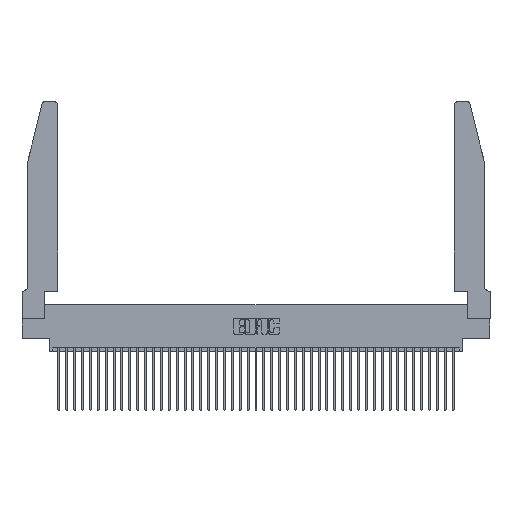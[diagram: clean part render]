
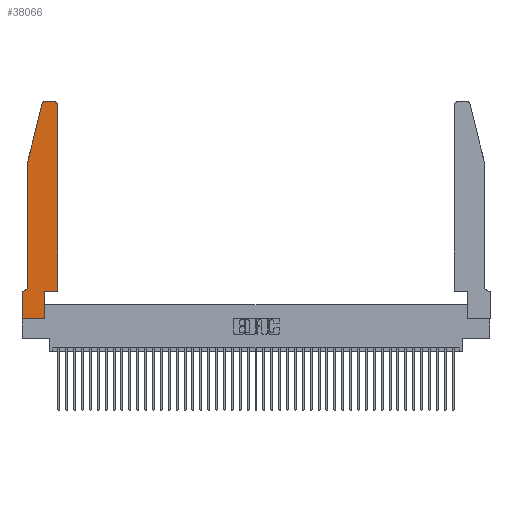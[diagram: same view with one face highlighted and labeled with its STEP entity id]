
A CAD part, top view. The second image highlights one B-rep face of the part: STEP entity #38066.
In plain terms, the highlighted planar face has unit normal (0, 0, 1).
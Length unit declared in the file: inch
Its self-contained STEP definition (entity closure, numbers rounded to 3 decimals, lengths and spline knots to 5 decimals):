
#344 = DIRECTION ( 'NONE',  ( 1., 0., 0. ) ) ;
#655 = VERTEX_POINT ( 'NONE', #27493 ) ;
#808 = VERTEX_POINT ( 'NONE', #23165 ) ;
#838 = CARTESIAN_POINT ( 'NONE',  ( 0.0055, 0.35, 0.37 ) ) ;
#1015 = EDGE_CURVE ( 'NONE', #15155, #16034, #19048, .T. ) ;
#1207 = CARTESIAN_POINT ( 'NONE',  ( 0.2605, 2.75, 0.37 ) ) ;
#1279 = VERTEX_POINT ( 'NONE', #5103 ) ;
#1773 = CARTESIAN_POINT ( 'NONE',  ( 0.284, 2.75, 0.37 ) ) ;
#2813 = EDGE_CURVE ( 'NONE', #16034, #808, #14678, .T. ) ;
#3134 = VERTEX_POINT ( 'NONE', #838 ) ;
#3527 = LINE ( 'NONE', #32728, #4634 ) ;
#4035 = CARTESIAN_POINT ( 'NONE',  ( 0.4205, 2.72, 0.37 ) ) ;
#4056 = LINE ( 'NONE', #37252, #11062 ) ;
#4232 = VERTEX_POINT ( 'NONE', #1773 ) ;
#4634 = VECTOR ( 'NONE', #9060, 39.37008 ) ;
#5055 = ORIENTED_EDGE ( 'NONE', *, *, #42771, .T. ) ;
#5103 = CARTESIAN_POINT ( 'NONE',  ( 0.4505, 0.35, 0.37 ) ) ;
#5328 = AXIS2_PLACEMENT_3D ( 'NONE', #7222, #20881, #344 ) ;
#6149 = VECTOR ( 'NONE', #42377, 39.37008 ) ;
#7222 = CARTESIAN_POINT ( 'NONE',  ( 0., 0.35, 0.37 ) ) ;
#7456 = EDGE_CURVE ( 'NONE', #41823, #11102, #25633, .T. ) ;
#7550 = DIRECTION ( 'NONE',  ( 1., 0., 0. ) ) ;
#8042 = AXIS2_PLACEMENT_3D ( 'NONE', #4035, #27740, #7550 ) ;
#8118 = CARTESIAN_POINT ( 'NONE',  ( 0.2865, 0.35, 0.37 ) ) ;
#8283 = FACE_OUTER_BOUND ( 'NONE', #43312, .T. ) ;
#8326 = ORIENTED_EDGE ( 'NONE', *, *, #26272, .T. ) ;
#8571 = ORIENTED_EDGE ( 'NONE', *, *, #2813, .T. ) ;
#9060 = DIRECTION ( 'NONE',  ( 0., 1., 0. ) ) ;
#9085 = CARTESIAN_POINT ( 'NONE',  ( 0., 0., 0.37 ) ) ;
#9821 = LINE ( 'NONE', #21708, #35583 ) ;
#10129 = VERTEX_POINT ( 'NONE', #19170 ) ;
#10695 = CARTESIAN_POINT ( 'NONE',  ( 0.2865, 0., 0.37 ) ) ;
#11062 = VECTOR ( 'NONE', #40607, 39.37008 ) ;
#11102 = VERTEX_POINT ( 'NONE', #10695 ) ;
#12475 = LINE ( 'NONE', #8118, #13531 ) ;
#13531 = VECTOR ( 'NONE', #41724, 39.37008 ) ;
#14416 = ORIENTED_EDGE ( 'NONE', *, *, #18797, .T. ) ;
#14678 = LINE ( 'NONE', #36544, #41377 ) ;
#15155 = VERTEX_POINT ( 'NONE', #40575 ) ;
#15384 = EDGE_CURVE ( 'NONE', #11102, #655, #12475, .T. ) ;
#15689 = DIRECTION ( 'NONE',  ( 0., 0., -1. ) ) ;
#16034 = VERTEX_POINT ( 'NONE', #35415 ) ;
#18371 = CARTESIAN_POINT ( 'NONE',  ( 0.284, 2.72, 0.37 ) ) ;
#18488 = ORIENTED_EDGE ( 'NONE', *, *, #7456, .T. ) ;
#18797 = EDGE_CURVE ( 'NONE', #4232, #15155, #30576, .T. ) ;
#18809 = EDGE_CURVE ( 'NONE', #23885, #4232, #21705, .T. ) ;
#19048 = LINE ( 'NONE', #39644, #43496 ) ;
#19170 = CARTESIAN_POINT ( 'NONE',  ( 0., 0.35, 0.37 ) ) ;
#20881 = DIRECTION ( 'NONE',  ( 0., 0., 1. ) ) ;
#21597 = ORIENTED_EDGE ( 'NONE', *, *, #15384, .T. ) ;
#21697 = DIRECTION ( 'NONE',  ( 1., 0., 0. ) ) ;
#21705 = LINE ( 'NONE', #1207, #29538 ) ;
#21708 = CARTESIAN_POINT ( 'NONE',  ( 0.0755, 0.35, 0.37 ) ) ;
#21833 = EDGE_CURVE ( 'NONE', #808, #3134, #27213, .T. ) ;
#22579 = ORIENTED_EDGE ( 'NONE', *, *, #32220, .T. ) ;
#23165 = CARTESIAN_POINT ( 'NONE',  ( 0.0755, 0.42, 0.37 ) ) ;
#23885 = VERTEX_POINT ( 'NONE', #39431 ) ;
#25067 = DIRECTION ( 'NONE',  ( -1., 0., 0. ) ) ;
#25213 = LINE ( 'NONE', #42238, #6149 ) ;
#25633 = LINE ( 'NONE', #38494, #34489 ) ;
#25707 = ORIENTED_EDGE ( 'NONE', *, *, #31964, .T. ) ;
#26256 = ORIENTED_EDGE ( 'NONE', *, *, #21833, .T. ) ;
#26272 = EDGE_CURVE ( 'NONE', #10129, #41823, #25213, .T. ) ;
#27213 = CIRCLE ( 'NONE', #32574, 0.07 ) ;
#27493 = CARTESIAN_POINT ( 'NONE',  ( 0.2865, 0.35, 0.37 ) ) ;
#27740 = DIRECTION ( 'NONE',  ( 0., 0., 1. ) ) ;
#28253 = DIRECTION ( 'NONE',  ( -1., 0., 0. ) ) ;
#29538 = VECTOR ( 'NONE', #28253, 39.37008 ) ;
#29832 = DIRECTION ( 'NONE',  ( 0., -1., 0. ) ) ;
#30576 = CIRCLE ( 'NONE', #42296, 0.03 ) ;
#30964 = DIRECTION ( 'NONE',  ( -0.239, -0.971, 0. ) ) ;
#31203 = ORIENTED_EDGE ( 'NONE', *, *, #18809, .T. ) ;
#31964 = EDGE_CURVE ( 'NONE', #1279, #41457, #3527, .T. ) ;
#32220 = EDGE_CURVE ( 'NONE', #655, #1279, #4056, .T. ) ;
#32574 = AXIS2_PLACEMENT_3D ( 'NONE', #35705, #15689, #39066 ) ;
#32728 = CARTESIAN_POINT ( 'NONE',  ( 0.4505, 0.35, 0.37 ) ) ;
#34323 = ORIENTED_EDGE ( 'NONE', *, *, #1015, .T. ) ;
#34489 = VECTOR ( 'NONE', #41820, 39.37008 ) ;
#34770 = EDGE_CURVE ( 'NONE', #3134, #10129, #9821, .T. ) ;
#35415 = CARTESIAN_POINT ( 'NONE',  ( 0.0755, 2., 0.37 ) ) ;
#35583 = VECTOR ( 'NONE', #25067, 39.37008 ) ;
#35705 = CARTESIAN_POINT ( 'NONE',  ( 0.0055, 0.42, 0.37 ) ) ;
#36544 = CARTESIAN_POINT ( 'NONE',  ( 0.0755, 2., 0.37 ) ) ;
#37252 = CARTESIAN_POINT ( 'NONE',  ( 0.4505, 0.35, 0.37 ) ) ;
#38066 = ADVANCED_FACE ( 'NONE', ( #8283 ), #40717, .T. ) ;
#38494 = CARTESIAN_POINT ( 'NONE',  ( 0., 0., 0.37 ) ) ;
#39066 = DIRECTION ( 'NONE',  ( -1., 0., 0. ) ) ;
#39431 = CARTESIAN_POINT ( 'NONE',  ( 0.4205, 2.75, 0.37 ) ) ;
#39644 = CARTESIAN_POINT ( 'NONE',  ( 0.0755, 2., 0.37 ) ) ;
#40575 = CARTESIAN_POINT ( 'NONE',  ( 0.25487, 2.72718, 0.37 ) ) ;
#40607 = DIRECTION ( 'NONE',  ( 1., 0., 0. ) ) ;
#40684 = CARTESIAN_POINT ( 'NONE',  ( 0.4505, 2.72, 0.37 ) ) ;
#40717 = PLANE ( 'NONE',  #5328 ) ;
#40884 = ORIENTED_EDGE ( 'NONE', *, *, #34770, .T. ) ;
#41377 = VECTOR ( 'NONE', #29832, 39.37008 ) ;
#41457 = VERTEX_POINT ( 'NONE', #40684 ) ;
#41676 = DIRECTION ( 'NONE',  ( 0., 0., 1. ) ) ;
#41724 = DIRECTION ( 'NONE',  ( 0., 1., 0. ) ) ;
#41820 = DIRECTION ( 'NONE',  ( 1., 0., 0. ) ) ;
#41823 = VERTEX_POINT ( 'NONE', #9085 ) ;
#42238 = CARTESIAN_POINT ( 'NONE',  ( 0., 0., 0.37 ) ) ;
#42296 = AXIS2_PLACEMENT_3D ( 'NONE', #18371, #41676, #21697 ) ;
#42377 = DIRECTION ( 'NONE',  ( 0., -1., 0. ) ) ;
#42771 = EDGE_CURVE ( 'NONE', #41457, #23885, #43002, .T. ) ;
#43002 = CIRCLE ( 'NONE', #8042, 0.03 ) ;
#43312 = EDGE_LOOP ( 'NONE', ( #31203, #14416, #34323, #8571, #26256, #40884, #8326, #18488, #21597, #22579, #25707, #5055 ) ) ;
#43496 = VECTOR ( 'NONE', #30964, 39.37008 ) ;
